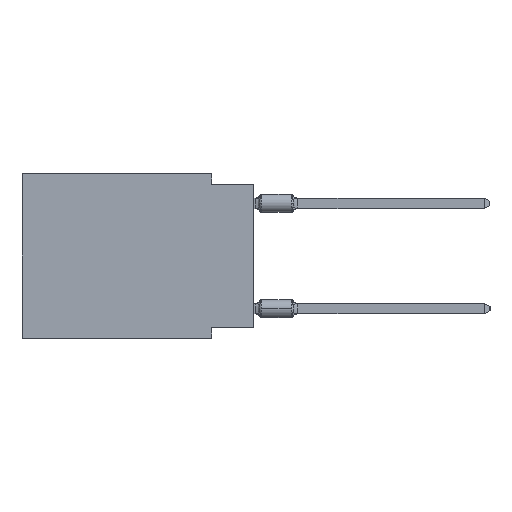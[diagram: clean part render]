
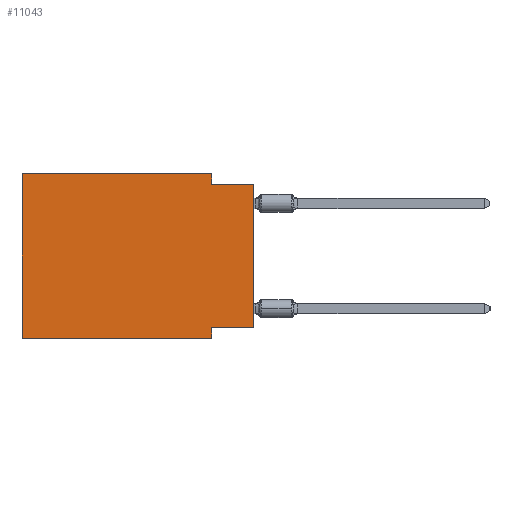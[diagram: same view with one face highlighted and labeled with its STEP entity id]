
A CAD part, left-side view. The second image highlights one B-rep face of the part: STEP entity #11043.
In plain terms, the highlighted planar face has unit normal (-1, 0, 0).
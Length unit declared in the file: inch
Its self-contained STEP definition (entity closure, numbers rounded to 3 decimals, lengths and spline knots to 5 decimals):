
#2355 = LINE ( 'NONE', #22685, #34922 ) ;
#2456 = CARTESIAN_POINT ( 'NONE',  ( 0., 0., -0.025 ) ) ;
#2789 = ORIENTED_EDGE ( 'NONE', *, *, #10769, .F. ) ;
#3271 = EDGE_CURVE ( 'NONE', #11658, #33146, #14729, .T. ) ;
#7202 = ORIENTED_EDGE ( 'NONE', *, *, #8637, .T. ) ;
#7883 = CARTESIAN_POINT ( 'NONE',  ( 0., 0.1, 0. ) ) ;
#8143 = DIRECTION ( 'NONE',  ( 0., 0., 1. ) ) ;
#8518 = LINE ( 'NONE', #20319, #31592 ) ;
#8637 = EDGE_CURVE ( 'NONE', #24862, #37232, #10448, .T. ) ;
#9503 = CARTESIAN_POINT ( 'NONE',  ( 0., 0.55, -0.39 ) ) ;
#9932 = VECTOR ( 'NONE', #19956, 39.37008 ) ;
#10448 = LINE ( 'NONE', #16450, #24532 ) ;
#10769 = EDGE_CURVE ( 'NONE', #28608, #35023, #26187, .T. ) ;
#11043 = ADVANCED_FACE ( 'NONE', ( #19740 ), #13743, .F. ) ;
#11188 = DIRECTION ( 'NONE',  ( 0., 0., -1. ) ) ;
#11380 = LINE ( 'NONE', #20084, #33502 ) ;
#11658 = VERTEX_POINT ( 'NONE', #25497 ) ;
#12578 = EDGE_CURVE ( 'NONE', #28608, #33146, #19376, .T. ) ;
#13159 = EDGE_CURVE ( 'NONE', #35023, #37232, #11380, .T. ) ;
#13360 = CARTESIAN_POINT ( 'NONE',  ( 0., 0.55, 0. ) ) ;
#13575 = CARTESIAN_POINT ( 'NONE',  ( 0., 0.55, 0. ) ) ;
#13743 = PLANE ( 'NONE',  #17884 ) ;
#14668 = VERTEX_POINT ( 'NONE', #7883 ) ;
#14729 = LINE ( 'NONE', #32303, #9932 ) ;
#15558 = CARTESIAN_POINT ( 'NONE',  ( 0., 0.55, 0. ) ) ;
#16450 = CARTESIAN_POINT ( 'NONE',  ( 0., 0.55, -0.39 ) ) ;
#16480 = LINE ( 'NONE', #13575, #33690 ) ;
#17497 = VERTEX_POINT ( 'NONE', #15558 ) ;
#17884 = AXIS2_PLACEMENT_3D ( 'NONE', #13360, #19356, #22263 ) ;
#18091 = ORIENTED_EDGE ( 'NONE', *, *, #26460, .F. ) ;
#19356 = DIRECTION ( 'NONE',  ( 1., 0., 0. ) ) ;
#19376 = LINE ( 'NONE', #31156, #36566 ) ;
#19740 = FACE_OUTER_BOUND ( 'NONE', #36730, .T. ) ;
#19956 = DIRECTION ( 'NONE',  ( 0., -1., 0. ) ) ;
#20084 = CARTESIAN_POINT ( 'NONE',  ( 0., 0.1, -0.39 ) ) ;
#20319 = CARTESIAN_POINT ( 'NONE',  ( 0., 0.1, 0. ) ) ;
#20461 = CARTESIAN_POINT ( 'NONE',  ( 0., 0.1, -0.39 ) ) ;
#21545 = CARTESIAN_POINT ( 'NONE',  ( 0., 0., -0.365 ) ) ;
#21557 = VECTOR ( 'NONE', #25614, 39.37008 ) ;
#22263 = DIRECTION ( 'NONE',  ( 0., 0., -1. ) ) ;
#22685 = CARTESIAN_POINT ( 'NONE',  ( 0., 0.55, 0. ) ) ;
#24532 = VECTOR ( 'NONE', #37274, 39.37008 ) ;
#24862 = VERTEX_POINT ( 'NONE', #9503 ) ;
#25497 = CARTESIAN_POINT ( 'NONE',  ( 0., 0.1, -0.025 ) ) ;
#25614 = DIRECTION ( 'NONE',  ( 0., 1., 0. ) ) ;
#26187 = LINE ( 'NONE', #34873, #21557 ) ;
#26460 = EDGE_CURVE ( 'NONE', #14668, #11658, #8518, .T. ) ;
#28453 = DIRECTION ( 'NONE',  ( 0., 0., 1. ) ) ;
#28608 = VERTEX_POINT ( 'NONE', #21545 ) ;
#31156 = CARTESIAN_POINT ( 'NONE',  ( 0., 0., 0. ) ) ;
#31477 = ORIENTED_EDGE ( 'NONE', *, *, #33873, .F. ) ;
#31592 = VECTOR ( 'NONE', #32108, 39.37008 ) ;
#31614 = ORIENTED_EDGE ( 'NONE', *, *, #12578, .T. ) ;
#32108 = DIRECTION ( 'NONE',  ( 0., 0., -1. ) ) ;
#32303 = CARTESIAN_POINT ( 'NONE',  ( 0., 0., -0.025 ) ) ;
#33146 = VERTEX_POINT ( 'NONE', #2456 ) ;
#33502 = VECTOR ( 'NONE', #11188, 39.37008 ) ;
#33690 = VECTOR ( 'NONE', #8143, 39.37008 ) ;
#33873 = EDGE_CURVE ( 'NONE', #24862, #17497, #16480, .T. ) ;
#34152 = ORIENTED_EDGE ( 'NONE', *, *, #3271, .F. ) ;
#34538 = ORIENTED_EDGE ( 'NONE', *, *, #35380, .F. ) ;
#34820 = CARTESIAN_POINT ( 'NONE',  ( 0., 0.1, -0.365 ) ) ;
#34873 = CARTESIAN_POINT ( 'NONE',  ( 0., 0., -0.365 ) ) ;
#34922 = VECTOR ( 'NONE', #38105, 39.37008 ) ;
#35023 = VERTEX_POINT ( 'NONE', #34820 ) ;
#35380 = EDGE_CURVE ( 'NONE', #17497, #14668, #2355, .T. ) ;
#36262 = ORIENTED_EDGE ( 'NONE', *, *, #13159, .F. ) ;
#36566 = VECTOR ( 'NONE', #28453, 39.37008 ) ;
#36730 = EDGE_LOOP ( 'NONE', ( #31614, #34152, #18091, #34538, #31477, #7202, #36262, #2789 ) ) ;
#37232 = VERTEX_POINT ( 'NONE', #20461 ) ;
#37274 = DIRECTION ( 'NONE',  ( 0., -1., 0. ) ) ;
#38105 = DIRECTION ( 'NONE',  ( 0., -1., 0. ) ) ;
